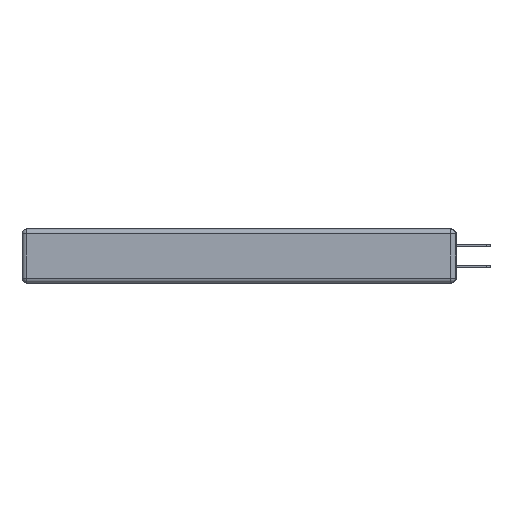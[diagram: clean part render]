
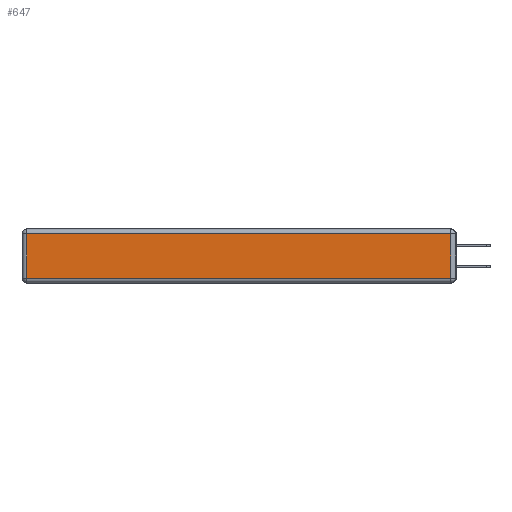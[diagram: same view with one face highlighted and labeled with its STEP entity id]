
A CAD part, left-side view. The second image highlights one B-rep face of the part: STEP entity #647.
In plain terms, the highlighted planar face has unit normal (-1, 0, 0).
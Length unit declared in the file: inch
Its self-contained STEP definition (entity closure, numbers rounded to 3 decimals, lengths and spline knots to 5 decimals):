
#133 = EDGE_CURVE ( 'NONE', #24255, #1835, #4963, .T. ) ;
#647 = ADVANCED_FACE ( 'NONE', ( #12781 ), #22558, .T. ) ;
#941 = CARTESIAN_POINT ( 'NONE',  ( 0., 0., -0.313 ) ) ;
#1038 = CARTESIAN_POINT ( 'NONE',  ( 0., 2.72, -0.343 ) ) ;
#1464 = ORIENTED_EDGE ( 'NONE', *, *, #19499, .T. ) ;
#1537 = VERTEX_POINT ( 'NONE', #10273 ) ;
#1835 = VERTEX_POINT ( 'NONE', #18105 ) ;
#3030 = CARTESIAN_POINT ( 'NONE',  ( 0., 0., -0.343 ) ) ;
#3211 = DIRECTION ( 'NONE',  ( -1., 0., 0. ) ) ;
#4911 = DIRECTION ( 'NONE',  ( 0., 0., 1. ) ) ;
#4963 = LINE ( 'NONE', #1038, #24905 ) ;
#5354 = LINE ( 'NONE', #11974, #15039 ) ;
#6854 = CARTESIAN_POINT ( 'NONE',  ( 0., 2.72, -0.03 ) ) ;
#7044 = CARTESIAN_POINT ( 'NONE',  ( 0., 0.03, -0.313 ) ) ;
#9502 = EDGE_CURVE ( 'NONE', #1835, #21133, #12762, .T. ) ;
#10273 = CARTESIAN_POINT ( 'NONE',  ( 0., 0.03, -0.03 ) ) ;
#10444 = VECTOR ( 'NONE', #16862, 39.37008 ) ;
#11091 = CARTESIAN_POINT ( 'NONE',  ( 0., 0.03, -0.343 ) ) ;
#11974 = CARTESIAN_POINT ( 'NONE',  ( 0., 2.75, -0.03 ) ) ;
#12550 = DIRECTION ( 'NONE',  ( 0., 0., -1. ) ) ;
#12762 = LINE ( 'NONE', #941, #17607 ) ;
#12781 = FACE_OUTER_BOUND ( 'NONE', #13086, .T. ) ;
#13086 = EDGE_LOOP ( 'NONE', ( #22187, #1464, #14305, #18937 ) ) ;
#14305 = ORIENTED_EDGE ( 'NONE', *, *, #19235, .T. ) ;
#15039 = VECTOR ( 'NONE', #22015, 39.37008 ) ;
#16862 = DIRECTION ( 'NONE',  ( 0., 0., 1. ) ) ;
#17607 = VECTOR ( 'NONE', #20291, 39.37008 ) ;
#18105 = CARTESIAN_POINT ( 'NONE',  ( 0., 2.72, -0.313 ) ) ;
#18937 = ORIENTED_EDGE ( 'NONE', *, *, #133, .T. ) ;
#19235 = EDGE_CURVE ( 'NONE', #1537, #24255, #5354, .T. ) ;
#19499 = EDGE_CURVE ( 'NONE', #21133, #1537, #24070, .T. ) ;
#20291 = DIRECTION ( 'NONE',  ( 0., -1., 0. ) ) ;
#21133 = VERTEX_POINT ( 'NONE', #7044 ) ;
#22015 = DIRECTION ( 'NONE',  ( 0., 1., 0. ) ) ;
#22187 = ORIENTED_EDGE ( 'NONE', *, *, #9502, .T. ) ;
#22558 = PLANE ( 'NONE',  #24028 ) ;
#24028 = AXIS2_PLACEMENT_3D ( 'NONE', #3030, #3211, #4911 ) ;
#24070 = LINE ( 'NONE', #11091, #10444 ) ;
#24255 = VERTEX_POINT ( 'NONE', #6854 ) ;
#24905 = VECTOR ( 'NONE', #12550, 39.37008 ) ;
